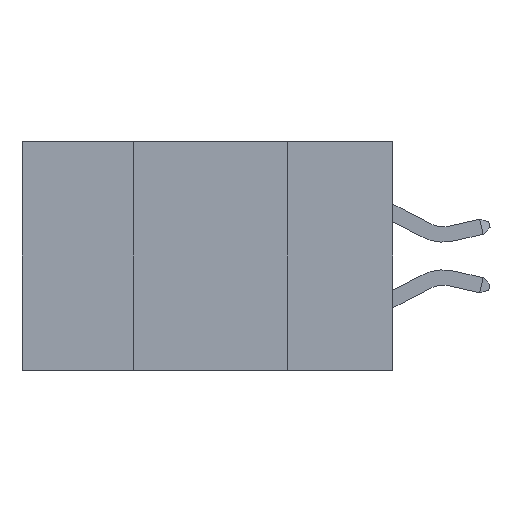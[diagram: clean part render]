
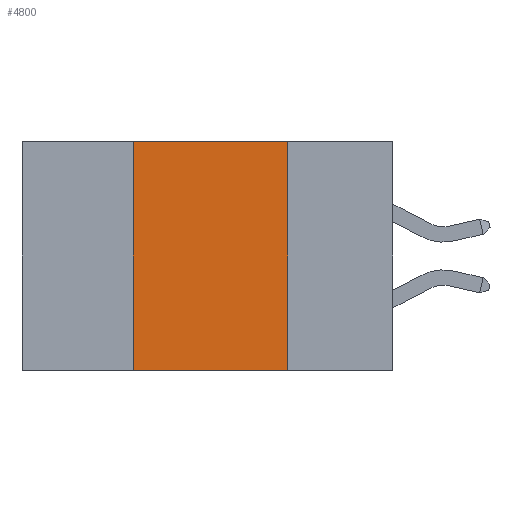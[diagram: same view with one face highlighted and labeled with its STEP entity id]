
A CAD part, left-side view. The second image highlights one B-rep face of the part: STEP entity #4800.
In plain terms, the highlighted planar face has unit normal (-1, 0, 0).
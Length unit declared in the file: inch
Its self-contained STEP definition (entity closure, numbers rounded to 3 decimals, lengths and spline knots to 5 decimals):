
#5 = PLANE ( 'NONE',  #2214 ) ;
#78 = CARTESIAN_POINT ( 'NONE',  ( 0., 0.6, 0. ) ) ;
#80 = VERTEX_POINT ( 'NONE', #3490 ) ;
#197 = LINE ( 'NONE', #5009, #9899 ) ;
#344 = LINE ( 'NONE', #2620, #2686 ) ;
#374 = EDGE_CURVE ( 'NONE', #1266, #2418, #3755, .T. ) ;
#987 = CARTESIAN_POINT ( 'NONE',  ( 0., 0.42, -0.37 ) ) ;
#1154 = VECTOR ( 'NONE', #8179, 39.37008 ) ;
#1266 = VERTEX_POINT ( 'NONE', #987 ) ;
#1467 = EDGE_CURVE ( 'NONE', #1266, #80, #197, .T. ) ;
#2214 = AXIS2_PLACEMENT_3D ( 'NONE', #78, #9916, #10532 ) ;
#2233 = VECTOR ( 'NONE', #10009, 39.37008 ) ;
#2410 = EDGE_CURVE ( 'NONE', #2418, #9031, #344, .T. ) ;
#2418 = VERTEX_POINT ( 'NONE', #5975 ) ;
#2528 = LINE ( 'NONE', #10047, #2233 ) ;
#2620 = CARTESIAN_POINT ( 'NONE',  ( 0., 0.6, 0. ) ) ;
#2686 = VECTOR ( 'NONE', #4959, 39.37008 ) ;
#3250 = CARTESIAN_POINT ( 'NONE',  ( 0., 0.42, 0. ) ) ;
#3490 = CARTESIAN_POINT ( 'NONE',  ( 0., 0.17, -0.37 ) ) ;
#3755 = LINE ( 'NONE', #3250, #1154 ) ;
#4479 = EDGE_CURVE ( 'NONE', #9031, #80, #2528, .T. ) ;
#4800 = ADVANCED_FACE ( 'NONE', ( #10956 ), #5, .F. ) ;
#4959 = DIRECTION ( 'NONE',  ( 0., -1., 0. ) ) ;
#5009 = CARTESIAN_POINT ( 'NONE',  ( 0., 0.6, -0.37 ) ) ;
#5975 = CARTESIAN_POINT ( 'NONE',  ( 0., 0.42, 0. ) ) ;
#8052 = DIRECTION ( 'NONE',  ( 0., -1., 0. ) ) ;
#8179 = DIRECTION ( 'NONE',  ( 0., 0., 1. ) ) ;
#8222 = CARTESIAN_POINT ( 'NONE',  ( 0., 0.17, 0. ) ) ;
#8721 = EDGE_LOOP ( 'NONE', ( #11773, #11546, #9049, #8774 ) ) ;
#8774 = ORIENTED_EDGE ( 'NONE', *, *, #1467, .T. ) ;
#9031 = VERTEX_POINT ( 'NONE', #8222 ) ;
#9049 = ORIENTED_EDGE ( 'NONE', *, *, #374, .F. ) ;
#9899 = VECTOR ( 'NONE', #8052, 39.37008 ) ;
#9916 = DIRECTION ( 'NONE',  ( 1., 0., 0. ) ) ;
#10009 = DIRECTION ( 'NONE',  ( 0., 0., -1. ) ) ;
#10047 = CARTESIAN_POINT ( 'NONE',  ( 0., 0.17, 0. ) ) ;
#10532 = DIRECTION ( 'NONE',  ( 0., 0., -1. ) ) ;
#10956 = FACE_OUTER_BOUND ( 'NONE', #8721, .T. ) ;
#11546 = ORIENTED_EDGE ( 'NONE', *, *, #2410, .F. ) ;
#11773 = ORIENTED_EDGE ( 'NONE', *, *, #4479, .F. ) ;
